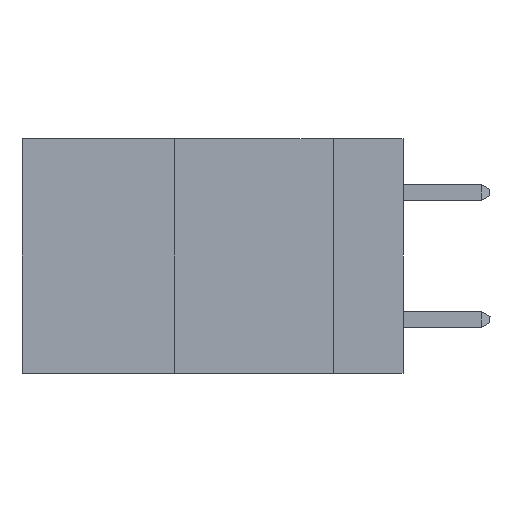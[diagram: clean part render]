
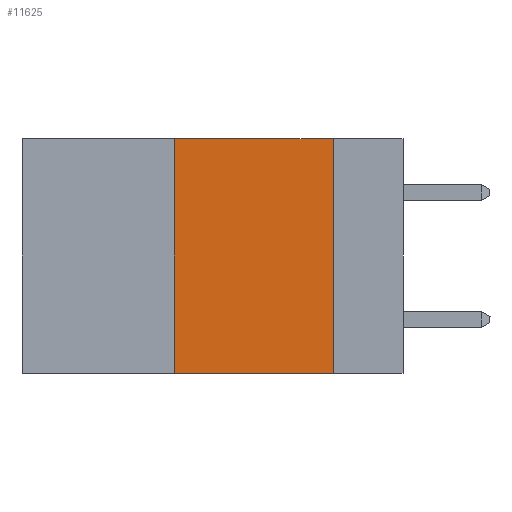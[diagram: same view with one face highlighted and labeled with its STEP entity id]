
A CAD part, left-side view. The second image highlights one B-rep face of the part: STEP entity #11625.
In plain terms, the highlighted planar face has unit normal (-1, 0, 0).
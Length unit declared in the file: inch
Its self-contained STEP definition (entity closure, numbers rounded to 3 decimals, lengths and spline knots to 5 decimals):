
#162 = VERTEX_POINT ( 'NONE', #11011 ) ;
#382 = DIRECTION ( 'NONE',  ( 0., 0., -1. ) ) ;
#785 = LINE ( 'NONE', #13990, #17249 ) ;
#1923 = VERTEX_POINT ( 'NONE', #14694 ) ;
#3313 = LINE ( 'NONE', #12516, #5891 ) ;
#3538 = CARTESIAN_POINT ( 'NONE',  ( 0., 0.6, -0.37 ) ) ;
#3586 = ORIENTED_EDGE ( 'NONE', *, *, #4805, .F. ) ;
#4595 = VERTEX_POINT ( 'NONE', #13647 ) ;
#4606 = DIRECTION ( 'NONE',  ( 1., 0., 0. ) ) ;
#4805 = EDGE_CURVE ( 'NONE', #7910, #162, #785, .T. ) ;
#4828 = CARTESIAN_POINT ( 'NONE',  ( 0., 0.36, 0. ) ) ;
#5040 = LINE ( 'NONE', #11589, #12297 ) ;
#5782 = EDGE_CURVE ( 'NONE', #162, #4595, #5040, .T. ) ;
#5891 = VECTOR ( 'NONE', #8464, 39.37008 ) ;
#6479 = EDGE_CURVE ( 'NONE', #1923, #7910, #3313, .T. ) ;
#7282 = CARTESIAN_POINT ( 'NONE',  ( 0., 0.6, 0. ) ) ;
#7361 = DIRECTION ( 'NONE',  ( 0., -1., 0. ) ) ;
#7712 = ORIENTED_EDGE ( 'NONE', *, *, #8807, .T. ) ;
#7910 = VERTEX_POINT ( 'NONE', #4828 ) ;
#8464 = DIRECTION ( 'NONE',  ( 0., 0., 1. ) ) ;
#8807 = EDGE_CURVE ( 'NONE', #1923, #4595, #14023, .T. ) ;
#9394 = EDGE_LOOP ( 'NONE', ( #13120, #3586, #10554, #7712 ) ) ;
#10554 = ORIENTED_EDGE ( 'NONE', *, *, #6479, .F. ) ;
#11011 = CARTESIAN_POINT ( 'NONE',  ( 0., 0.11, 0. ) ) ;
#11461 = DIRECTION ( 'NONE',  ( 0., -1., 0. ) ) ;
#11589 = CARTESIAN_POINT ( 'NONE',  ( 0., 0.11, 0. ) ) ;
#11625 = ADVANCED_FACE ( 'NONE', ( #13608 ), #16406, .F. ) ;
#12297 = VECTOR ( 'NONE', #13004, 39.37008 ) ;
#12516 = CARTESIAN_POINT ( 'NONE',  ( 0., 0.36, 0. ) ) ;
#13004 = DIRECTION ( 'NONE',  ( 0., 0., -1. ) ) ;
#13120 = ORIENTED_EDGE ( 'NONE', *, *, #5782, .F. ) ;
#13452 = AXIS2_PLACEMENT_3D ( 'NONE', #7282, #4606, #382 ) ;
#13608 = FACE_OUTER_BOUND ( 'NONE', #9394, .T. ) ;
#13647 = CARTESIAN_POINT ( 'NONE',  ( 0., 0.11, -0.37 ) ) ;
#13990 = CARTESIAN_POINT ( 'NONE',  ( 0., 0.6, 0. ) ) ;
#14023 = LINE ( 'NONE', #3538, #14662 ) ;
#14662 = VECTOR ( 'NONE', #7361, 39.37008 ) ;
#14694 = CARTESIAN_POINT ( 'NONE',  ( 0., 0.36, -0.37 ) ) ;
#16406 = PLANE ( 'NONE',  #13452 ) ;
#17249 = VECTOR ( 'NONE', #11461, 39.37008 ) ;
